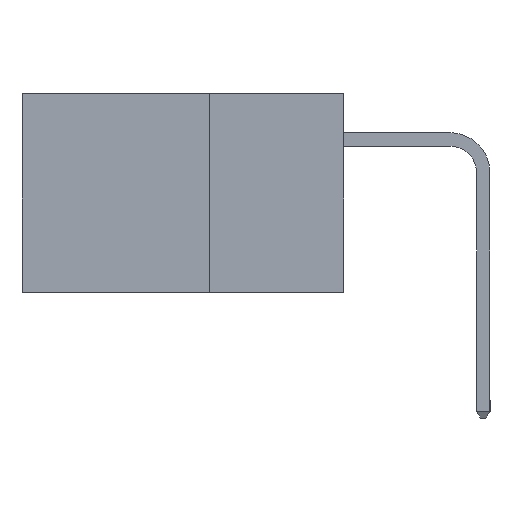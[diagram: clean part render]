
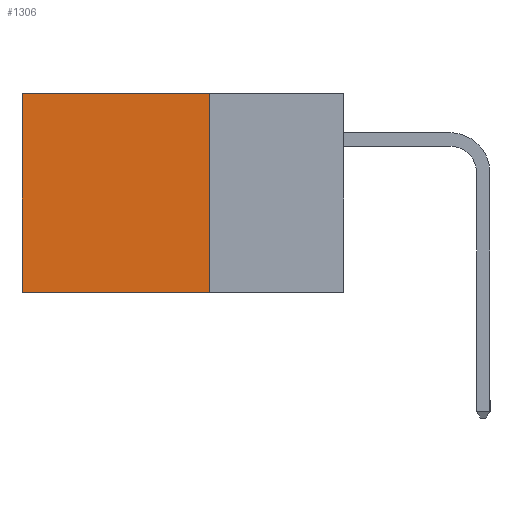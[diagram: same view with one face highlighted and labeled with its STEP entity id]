
A CAD part, left-side view. The second image highlights one B-rep face of the part: STEP entity #1306.
In plain terms, the highlighted planar face has unit normal (-1, 0, 0).
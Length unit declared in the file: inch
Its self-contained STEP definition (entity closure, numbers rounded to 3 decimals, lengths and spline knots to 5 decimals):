
#221 = LINE ( 'NONE', #8717, #9339 ) ;
#272 = VECTOR ( 'NONE', #2267, 39.37008 ) ;
#474 = DIRECTION ( 'NONE',  ( 0., 0., -1. ) ) ;
#1306 = ADVANCED_FACE ( 'NONE', ( #7115 ), #7554, .F. ) ;
#1678 = CARTESIAN_POINT ( 'NONE',  ( 0.2615, 0.6, -0.37 ) ) ;
#1733 = EDGE_LOOP ( 'NONE', ( #8690, #6511, #6333, #3748 ) ) ;
#2267 = DIRECTION ( 'NONE',  ( 0., 1., 0. ) ) ;
#2350 = CARTESIAN_POINT ( 'NONE',  ( 0.2615, 0.6, 0. ) ) ;
#3460 = DIRECTION ( 'NONE',  ( 0., 0., -1. ) ) ;
#3505 = LINE ( 'NONE', #15067, #272 ) ;
#3719 = CARTESIAN_POINT ( 'NONE',  ( 0.2615, 0.25, 0. ) ) ;
#3748 = ORIENTED_EDGE ( 'NONE', *, *, #4708, .T. ) ;
#4206 = VERTEX_POINT ( 'NONE', #7346 ) ;
#4597 = CARTESIAN_POINT ( 'NONE',  ( 0.2615, 0.25, -0.37 ) ) ;
#4708 = EDGE_CURVE ( 'NONE', #4206, #10626, #8841, .T. ) ;
#6035 = EDGE_CURVE ( 'NONE', #4206, #9997, #221, .T. ) ;
#6333 = ORIENTED_EDGE ( 'NONE', *, *, #6035, .F. ) ;
#6511 = ORIENTED_EDGE ( 'NONE', *, *, #9963, .F. ) ;
#6683 = CARTESIAN_POINT ( 'NONE',  ( 0.2615, 0.6, -0.37 ) ) ;
#7041 = EDGE_CURVE ( 'NONE', #10626, #14096, #11827, .T. ) ;
#7115 = FACE_OUTER_BOUND ( 'NONE', #1733, .T. ) ;
#7346 = CARTESIAN_POINT ( 'NONE',  ( 0.2615, 0.25, 0. ) ) ;
#7554 = PLANE ( 'NONE',  #7784 ) ;
#7784 = AXIS2_PLACEMENT_3D ( 'NONE', #4597, #8647, #3460 ) ;
#8386 = VECTOR ( 'NONE', #474, 39.37008 ) ;
#8457 = DIRECTION ( 'NONE',  ( 0., 1., 0. ) ) ;
#8647 = DIRECTION ( 'NONE',  ( 1., 0., 0. ) ) ;
#8690 = ORIENTED_EDGE ( 'NONE', *, *, #7041, .T. ) ;
#8717 = CARTESIAN_POINT ( 'NONE',  ( 0.2615, 0.25, -0.37 ) ) ;
#8777 = DIRECTION ( 'NONE',  ( 0., 0., -1. ) ) ;
#8841 = LINE ( 'NONE', #3719, #14194 ) ;
#9339 = VECTOR ( 'NONE', #8777, 39.37008 ) ;
#9963 = EDGE_CURVE ( 'NONE', #9997, #14096, #3505, .T. ) ;
#9997 = VERTEX_POINT ( 'NONE', #10549 ) ;
#10549 = CARTESIAN_POINT ( 'NONE',  ( 0.2615, 0.25, -0.37 ) ) ;
#10626 = VERTEX_POINT ( 'NONE', #2350 ) ;
#11827 = LINE ( 'NONE', #1678, #8386 ) ;
#14096 = VERTEX_POINT ( 'NONE', #6683 ) ;
#14194 = VECTOR ( 'NONE', #8457, 39.37008 ) ;
#15067 = CARTESIAN_POINT ( 'NONE',  ( 0.2615, 0.25, -0.37 ) ) ;
